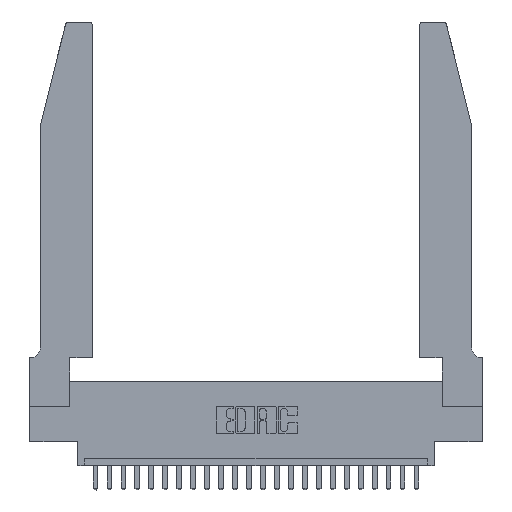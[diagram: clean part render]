
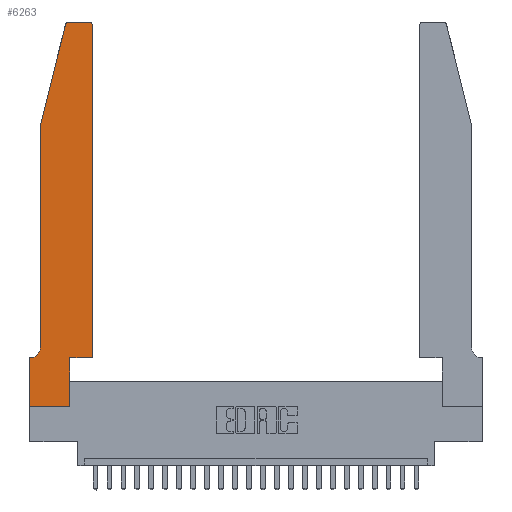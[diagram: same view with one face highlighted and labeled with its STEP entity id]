
A CAD part, top view. The second image highlights one B-rep face of the part: STEP entity #6263.
In plain terms, the highlighted planar face has unit normal (0, 0, 1).
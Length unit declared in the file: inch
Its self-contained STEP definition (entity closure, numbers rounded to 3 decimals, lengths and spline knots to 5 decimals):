
#28 = ORIENTED_EDGE ( 'NONE', *, *, #9581, .T. ) ;
#156 = ORIENTED_EDGE ( 'NONE', *, *, #23107, .T. ) ;
#382 = DIRECTION ( 'NONE',  ( 1., 0., 0. ) ) ;
#517 = EDGE_CURVE ( 'NONE', #20964, #9428, #5502, .T. ) ;
#621 = ORIENTED_EDGE ( 'NONE', *, *, #10142, .T. ) ;
#921 = DIRECTION ( 'NONE',  ( 0., 0., 1. ) ) ;
#938 = CARTESIAN_POINT ( 'NONE',  ( 0.4505, 0.35, 0.37 ) ) ;
#1329 = CARTESIAN_POINT ( 'NONE',  ( 0., 0., 0.37 ) ) ;
#1523 = CARTESIAN_POINT ( 'NONE',  ( 0., 0., 0.37 ) ) ;
#1560 = VECTOR ( 'NONE', #20626, 39.37008 ) ;
#1718 = VERTEX_POINT ( 'NONE', #1329 ) ;
#1841 = LINE ( 'NONE', #25337, #24279 ) ;
#3287 = CARTESIAN_POINT ( 'NONE',  ( 0., 0.35, 0.37 ) ) ;
#3504 = DIRECTION ( 'NONE',  ( 1., 0., 0. ) ) ;
#3520 = ORIENTED_EDGE ( 'NONE', *, *, #11575, .T. ) ;
#3602 = CARTESIAN_POINT ( 'NONE',  ( 0.0755, 2., 0.37 ) ) ;
#3890 = EDGE_CURVE ( 'NONE', #9428, #19742, #22688, .T. ) ;
#4035 = EDGE_CURVE ( 'NONE', #22652, #1718, #12567, .T. ) ;
#4129 = DIRECTION ( 'NONE',  ( -1., 0., 0. ) ) ;
#4334 = VERTEX_POINT ( 'NONE', #6566 ) ;
#4400 = DIRECTION ( 'NONE',  ( 0., 0., 1. ) ) ;
#4420 = AXIS2_PLACEMENT_3D ( 'NONE', #6493, #12436, #14207 ) ;
#5502 = CIRCLE ( 'NONE', #13062, 0.03 ) ;
#5846 = CARTESIAN_POINT ( 'NONE',  ( 0.0055, 0.35, 0.37 ) ) ;
#6141 = DIRECTION ( 'NONE',  ( 0., 1., 0. ) ) ;
#6210 = VECTOR ( 'NONE', #6141, 39.37008 ) ;
#6263 = ADVANCED_FACE ( 'NONE', ( #18619 ), #8458, .T. ) ;
#6449 = CARTESIAN_POINT ( 'NONE',  ( 0.0055, 0.42, 0.37 ) ) ;
#6493 = CARTESIAN_POINT ( 'NONE',  ( 0., 0.35, 0.37 ) ) ;
#6566 = CARTESIAN_POINT ( 'NONE',  ( 0.0755, 0.42, 0.37 ) ) ;
#6994 = CARTESIAN_POINT ( 'NONE',  ( 0.284, 2.75, 0.37 ) ) ;
#7233 = ORIENTED_EDGE ( 'NONE', *, *, #15311, .T. ) ;
#7573 = AXIS2_PLACEMENT_3D ( 'NONE', #22393, #921, #10754 ) ;
#7932 = DIRECTION ( 'NONE',  ( 0., 1., 0. ) ) ;
#8037 = CIRCLE ( 'NONE', #7573, 0.03 ) ;
#8458 = PLANE ( 'NONE',  #4420 ) ;
#8513 = ORIENTED_EDGE ( 'NONE', *, *, #517, .T. ) ;
#8524 = EDGE_CURVE ( 'NONE', #17135, #11411, #11471, .T. ) ;
#9428 = VERTEX_POINT ( 'NONE', #10809 ) ;
#9581 = EDGE_CURVE ( 'NONE', #19479, #22652, #1841, .T. ) ;
#10097 = EDGE_CURVE ( 'NONE', #1718, #17135, #18287, .T. ) ;
#10142 = EDGE_CURVE ( 'NONE', #4334, #19479, #20320, .T. ) ;
#10591 = DIRECTION ( 'NONE',  ( -1., 0., 0. ) ) ;
#10636 = LINE ( 'NONE', #22445, #14291 ) ;
#10754 = DIRECTION ( 'NONE',  ( 1., 0., 0. ) ) ;
#10809 = CARTESIAN_POINT ( 'NONE',  ( 0.4205, 2.75, 0.37 ) ) ;
#11042 = CARTESIAN_POINT ( 'NONE',  ( 0.2865, 0., 0.37 ) ) ;
#11411 = VERTEX_POINT ( 'NONE', #16535 ) ;
#11471 = LINE ( 'NONE', #24352, #6210 ) ;
#11575 = EDGE_CURVE ( 'NONE', #15747, #4334, #17254, .T. ) ;
#12121 = EDGE_LOOP ( 'NONE', ( #22845, #20823, #20329, #3520, #621, #28, #23569, #23085, #19697, #156, #7233, #8513 ) ) ;
#12251 = CARTESIAN_POINT ( 'NONE',  ( 0.4505, 0.35, 0.37 ) ) ;
#12436 = DIRECTION ( 'NONE',  ( 0., 0., 1. ) ) ;
#12567 = LINE ( 'NONE', #24017, #23280 ) ;
#13062 = AXIS2_PLACEMENT_3D ( 'NONE', #22223, #4400, #382 ) ;
#13561 = DIRECTION ( 'NONE',  ( -1., 0., 0. ) ) ;
#14207 = DIRECTION ( 'NONE',  ( 1., 0., 0. ) ) ;
#14291 = VECTOR ( 'NONE', #7932, 39.37008 ) ;
#14426 = DIRECTION ( 'NONE',  ( 1., 0., 0. ) ) ;
#15311 = EDGE_CURVE ( 'NONE', #22434, #20964, #10636, .T. ) ;
#15683 = AXIS2_PLACEMENT_3D ( 'NONE', #6449, #18376, #10591 ) ;
#15747 = VERTEX_POINT ( 'NONE', #25060 ) ;
#15970 = VECTOR ( 'NONE', #4129, 39.37008 ) ;
#16067 = DIRECTION ( 'NONE',  ( 0., -1., 0. ) ) ;
#16175 = CARTESIAN_POINT ( 'NONE',  ( 0.25487, 2.72718, 0.37 ) ) ;
#16535 = CARTESIAN_POINT ( 'NONE',  ( 0.2865, 0.35, 0.37 ) ) ;
#16705 = EDGE_CURVE ( 'NONE', #19742, #18333, #8037, .T. ) ;
#17131 = CARTESIAN_POINT ( 'NONE',  ( 0.4505, 2.72, 0.37 ) ) ;
#17135 = VERTEX_POINT ( 'NONE', #11042 ) ;
#17254 = LINE ( 'NONE', #18903, #1560 ) ;
#17405 = VECTOR ( 'NONE', #24992, 39.37008 ) ;
#18122 = EDGE_CURVE ( 'NONE', #18333, #15747, #22603, .T. ) ;
#18287 = LINE ( 'NONE', #1523, #19811 ) ;
#18333 = VERTEX_POINT ( 'NONE', #16175 ) ;
#18376 = DIRECTION ( 'NONE',  ( 0., 0., -1. ) ) ;
#18619 = FACE_OUTER_BOUND ( 'NONE', #12121, .T. ) ;
#18903 = CARTESIAN_POINT ( 'NONE',  ( 0.0755, 2., 0.37 ) ) ;
#19479 = VERTEX_POINT ( 'NONE', #5846 ) ;
#19697 = ORIENTED_EDGE ( 'NONE', *, *, #8524, .T. ) ;
#19742 = VERTEX_POINT ( 'NONE', #6994 ) ;
#19811 = VECTOR ( 'NONE', #3504, 39.37008 ) ;
#20320 = CIRCLE ( 'NONE', #15683, 0.07 ) ;
#20329 = ORIENTED_EDGE ( 'NONE', *, *, #18122, .T. ) ;
#20626 = DIRECTION ( 'NONE',  ( 0., -1., 0. ) ) ;
#20823 = ORIENTED_EDGE ( 'NONE', *, *, #16705, .T. ) ;
#20964 = VERTEX_POINT ( 'NONE', #17131 ) ;
#22223 = CARTESIAN_POINT ( 'NONE',  ( 0.4205, 2.72, 0.37 ) ) ;
#22393 = CARTESIAN_POINT ( 'NONE',  ( 0.284, 2.72, 0.37 ) ) ;
#22434 = VERTEX_POINT ( 'NONE', #12251 ) ;
#22445 = CARTESIAN_POINT ( 'NONE',  ( 0.4505, 0.35, 0.37 ) ) ;
#22603 = LINE ( 'NONE', #3602, #17405 ) ;
#22652 = VERTEX_POINT ( 'NONE', #3287 ) ;
#22676 = VECTOR ( 'NONE', #14426, 39.37008 ) ;
#22688 = LINE ( 'NONE', #25411, #15970 ) ;
#22845 = ORIENTED_EDGE ( 'NONE', *, *, #3890, .T. ) ;
#23085 = ORIENTED_EDGE ( 'NONE', *, *, #10097, .T. ) ;
#23107 = EDGE_CURVE ( 'NONE', #11411, #22434, #24550, .T. ) ;
#23280 = VECTOR ( 'NONE', #16067, 39.37008 ) ;
#23569 = ORIENTED_EDGE ( 'NONE', *, *, #4035, .T. ) ;
#24017 = CARTESIAN_POINT ( 'NONE',  ( 0., 0., 0.37 ) ) ;
#24279 = VECTOR ( 'NONE', #13561, 39.37008 ) ;
#24352 = CARTESIAN_POINT ( 'NONE',  ( 0.2865, 0.35, 0.37 ) ) ;
#24550 = LINE ( 'NONE', #938, #22676 ) ;
#24992 = DIRECTION ( 'NONE',  ( -0.239, -0.971, 0. ) ) ;
#25060 = CARTESIAN_POINT ( 'NONE',  ( 0.0755, 2., 0.37 ) ) ;
#25337 = CARTESIAN_POINT ( 'NONE',  ( 0.0755, 0.35, 0.37 ) ) ;
#25411 = CARTESIAN_POINT ( 'NONE',  ( 0.2605, 2.75, 0.37 ) ) ;
